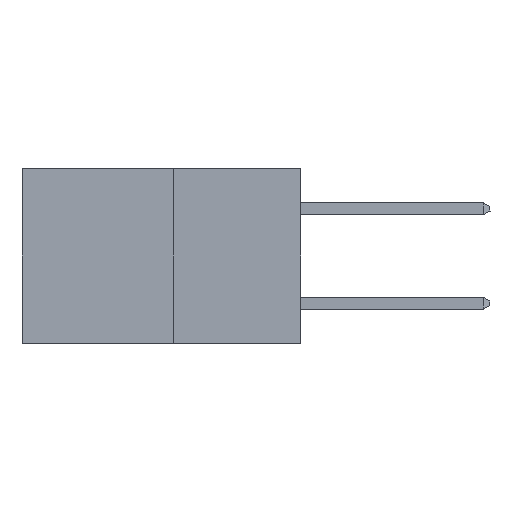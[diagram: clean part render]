
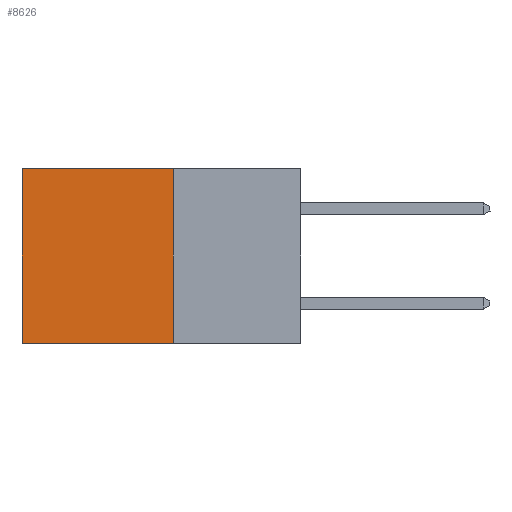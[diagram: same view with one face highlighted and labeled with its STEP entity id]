
A CAD part, left-side view. The second image highlights one B-rep face of the part: STEP entity #8626.
In plain terms, the highlighted planar face has unit normal (-1, 0, 0).
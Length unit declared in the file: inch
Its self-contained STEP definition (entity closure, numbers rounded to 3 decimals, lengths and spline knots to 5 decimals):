
#656 = ORIENTED_EDGE ( 'NONE', *, *, #8180, .F. ) ;
#2089 = ORIENTED_EDGE ( 'NONE', *, *, #5380, .T. ) ;
#2215 = CARTESIAN_POINT ( 'NONE',  ( 0.277, 0.59, -0.37 ) ) ;
#2491 = FACE_OUTER_BOUND ( 'NONE', #2955, .T. ) ;
#2955 = EDGE_LOOP ( 'NONE', ( #7046, #656, #7386, #2089 ) ) ;
#4298 = CARTESIAN_POINT ( 'NONE',  ( 0.277, 0.59, -0.37 ) ) ;
#4385 = VERTEX_POINT ( 'NONE', #4992 ) ;
#4992 = CARTESIAN_POINT ( 'NONE',  ( 0.277, 0.27, -0.37 ) ) ;
#5380 = EDGE_CURVE ( 'NONE', #7461, #10899, #10850, .T. ) ;
#6406 = CARTESIAN_POINT ( 'NONE',  ( 0.277, 0.59, 0. ) ) ;
#6425 = DIRECTION ( 'NONE',  ( 0., 0., -1. ) ) ;
#6436 = LINE ( 'NONE', #6717, #8816 ) ;
#6475 = DIRECTION ( 'NONE',  ( 1., 0., 0. ) ) ;
#6548 = PLANE ( 'NONE',  #12022 ) ;
#6717 = CARTESIAN_POINT ( 'NONE',  ( 0.277, 0.27, -0.37 ) ) ;
#7046 = ORIENTED_EDGE ( 'NONE', *, *, #12761, .T. ) ;
#7386 = ORIENTED_EDGE ( 'NONE', *, *, #11730, .F. ) ;
#7461 = VERTEX_POINT ( 'NONE', #9991 ) ;
#7514 = CARTESIAN_POINT ( 'NONE',  ( 0.277, 0.27, -0.37 ) ) ;
#7881 = DIRECTION ( 'NONE',  ( 0., 1., 0. ) ) ;
#8142 = VECTOR ( 'NONE', #7881, 39.37008 ) ;
#8180 = EDGE_CURVE ( 'NONE', #4385, #10402, #8276, .T. ) ;
#8276 = LINE ( 'NONE', #10683, #13270 ) ;
#8535 = VECTOR ( 'NONE', #9690, 39.37008 ) ;
#8626 = ADVANCED_FACE ( 'NONE', ( #2491 ), #6548, .F. ) ;
#8749 = DIRECTION ( 'NONE',  ( 0., 0., -1. ) ) ;
#8816 = VECTOR ( 'NONE', #8749, 39.37008 ) ;
#9690 = DIRECTION ( 'NONE',  ( 0., 0., -1. ) ) ;
#9991 = CARTESIAN_POINT ( 'NONE',  ( 0.277, 0.27, 0. ) ) ;
#10402 = VERTEX_POINT ( 'NONE', #4298 ) ;
#10512 = CARTESIAN_POINT ( 'NONE',  ( 0.277, 0.27, 0. ) ) ;
#10683 = CARTESIAN_POINT ( 'NONE',  ( 0.277, 0.27, -0.37 ) ) ;
#10772 = DIRECTION ( 'NONE',  ( 0., 1., 0. ) ) ;
#10850 = LINE ( 'NONE', #10512, #8142 ) ;
#10899 = VERTEX_POINT ( 'NONE', #6406 ) ;
#11549 = LINE ( 'NONE', #2215, #8535 ) ;
#11730 = EDGE_CURVE ( 'NONE', #7461, #4385, #6436, .T. ) ;
#12022 = AXIS2_PLACEMENT_3D ( 'NONE', #7514, #6475, #6425 ) ;
#12761 = EDGE_CURVE ( 'NONE', #10899, #10402, #11549, .T. ) ;
#13270 = VECTOR ( 'NONE', #10772, 39.37008 ) ;
